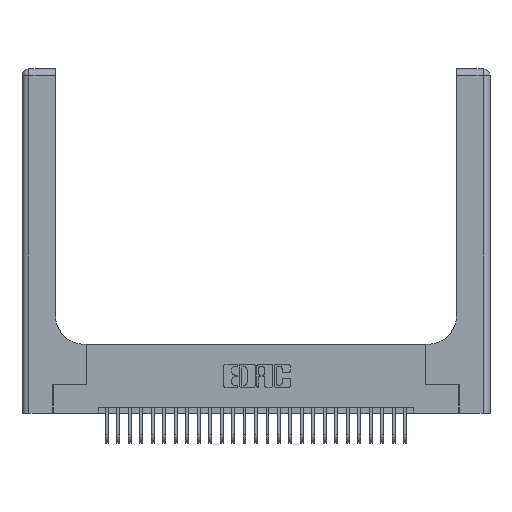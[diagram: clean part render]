
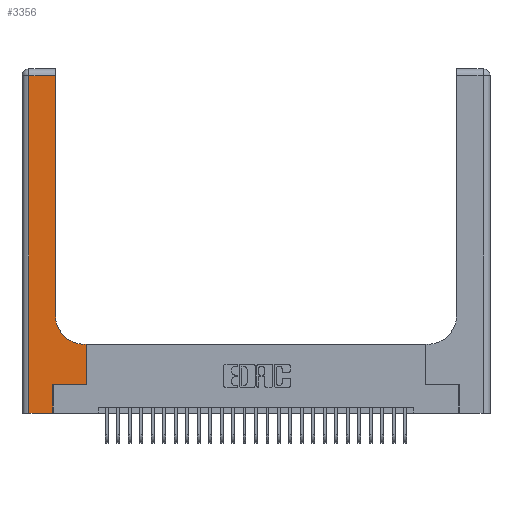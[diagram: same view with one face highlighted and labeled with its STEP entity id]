
A CAD part, top view. The second image highlights one B-rep face of the part: STEP entity #3356.
In plain terms, the highlighted planar face has unit normal (0, 0, 1).
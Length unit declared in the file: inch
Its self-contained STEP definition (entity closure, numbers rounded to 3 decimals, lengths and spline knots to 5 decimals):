
#152 = ORIENTED_EDGE ( 'NONE', *, *, #9684, .T. ) ;
#190 = EDGE_CURVE ( 'NONE', #2044, #9390, #6968, .T. ) ;
#1207 = ORIENTED_EDGE ( 'NONE', *, *, #14047, .T. ) ;
#1330 = VECTOR ( 'NONE', #9007, 39.37008 ) ;
#1758 = CARTESIAN_POINT ( 'NONE',  ( 0.2915, 3., 0.37 ) ) ;
#1813 = CARTESIAN_POINT ( 'NONE',  ( 0.269, 0.25, 0.37 ) ) ;
#2018 = EDGE_LOOP ( 'NONE', ( #13535, #4140, #25551, #152, #16556, #2170, #16359, #1207, #5405 ) ) ;
#2044 = VERTEX_POINT ( 'NONE', #18874 ) ;
#2170 = ORIENTED_EDGE ( 'NONE', *, *, #19964, .T. ) ;
#2260 = DIRECTION ( 'NONE',  ( 1., 0., 0. ) ) ;
#2372 = CARTESIAN_POINT ( 'NONE',  ( 0.269, 0.25, 0.37 ) ) ;
#2516 = CARTESIAN_POINT ( 'NONE',  ( 0.2915, 0.6, 0.37 ) ) ;
#3356 = ADVANCED_FACE ( 'NONE', ( #25059 ), #12335, .F. ) ;
#3654 = DIRECTION ( 'NONE',  ( 0., 0., -1. ) ) ;
#3860 = LINE ( 'NONE', #2372, #14624 ) ;
#3955 = DIRECTION ( 'NONE',  ( 0., 0., -1. ) ) ;
#4044 = DIRECTION ( 'NONE',  ( 0., -1., 0. ) ) ;
#4140 = ORIENTED_EDGE ( 'NONE', *, *, #23266, .T. ) ;
#5179 = LINE ( 'NONE', #14684, #26443 ) ;
#5287 = VERTEX_POINT ( 'NONE', #12602 ) ;
#5405 = ORIENTED_EDGE ( 'NONE', *, *, #15931, .T. ) ;
#5995 = AXIS2_PLACEMENT_3D ( 'NONE', #16468, #3654, #18598 ) ;
#6313 = VECTOR ( 'NONE', #21131, 39.37008 ) ;
#6968 = LINE ( 'NONE', #21126, #6313 ) ;
#9007 = DIRECTION ( 'NONE',  ( -1., 0., 0. ) ) ;
#9390 = VERTEX_POINT ( 'NONE', #22518 ) ;
#9440 = VERTEX_POINT ( 'NONE', #22958 ) ;
#9534 = DIRECTION ( 'NONE',  ( -1., 0., 0. ) ) ;
#9684 = EDGE_CURVE ( 'NONE', #12507, #16370, #10683, .T. ) ;
#10683 = LINE ( 'NONE', #25713, #26874 ) ;
#11013 = AXIS2_PLACEMENT_3D ( 'NONE', #16749, #3955, #18903 ) ;
#12335 = PLANE ( 'NONE',  #11013 ) ;
#12507 = VERTEX_POINT ( 'NONE', #18781 ) ;
#12533 = DIRECTION ( 'NONE',  ( 0., 1., 0. ) ) ;
#12602 = CARTESIAN_POINT ( 'NONE',  ( 0.06, 2.94, 0.37 ) ) ;
#12833 = LINE ( 'NONE', #2516, #1330 ) ;
#13219 = CARTESIAN_POINT ( 'NONE',  ( 0.2915, 2.94, 0.37 ) ) ;
#13535 = ORIENTED_EDGE ( 'NONE', *, *, #23711, .T. ) ;
#13866 = CARTESIAN_POINT ( 'NONE',  ( 0.2915, 0.85, 0.37 ) ) ;
#14047 = EDGE_CURVE ( 'NONE', #9390, #9440, #12833, .T. ) ;
#14624 = VECTOR ( 'NONE', #23636, 39.37008 ) ;
#14684 = CARTESIAN_POINT ( 'NONE',  ( 0.269, 0., 0.37 ) ) ;
#15686 = CIRCLE ( 'NONE', #5995, 0.25 ) ;
#15772 = VECTOR ( 'NONE', #9534, 39.37008 ) ;
#15931 = EDGE_CURVE ( 'NONE', #9440, #26290, #15686, .T. ) ;
#16359 = ORIENTED_EDGE ( 'NONE', *, *, #190, .T. ) ;
#16370 = VERTEX_POINT ( 'NONE', #24286 ) ;
#16441 = LINE ( 'NONE', #20114, #15772 ) ;
#16468 = CARTESIAN_POINT ( 'NONE',  ( 0.5415, 0.85, 0.37 ) ) ;
#16556 = ORIENTED_EDGE ( 'NONE', *, *, #20373, .T. ) ;
#16749 = CARTESIAN_POINT ( 'NONE',  ( 0., 3., 0.37 ) ) ;
#17307 = EDGE_CURVE ( 'NONE', #5287, #12507, #21218, .T. ) ;
#18598 = DIRECTION ( 'NONE',  ( 1., 0., 0. ) ) ;
#18781 = CARTESIAN_POINT ( 'NONE',  ( 0.06, 0., 0.37 ) ) ;
#18874 = CARTESIAN_POINT ( 'NONE',  ( 0.5585, 0.25, 0.37 ) ) ;
#18903 = DIRECTION ( 'NONE',  ( -1., 0., 0. ) ) ;
#19777 = VERTEX_POINT ( 'NONE', #1813 ) ;
#19964 = EDGE_CURVE ( 'NONE', #19777, #2044, #3860, .T. ) ;
#20114 = CARTESIAN_POINT ( 'NONE',  ( 0., 2.94, 0.37 ) ) ;
#20373 = EDGE_CURVE ( 'NONE', #16370, #19777, #5179, .T. ) ;
#21126 = CARTESIAN_POINT ( 'NONE',  ( 0.5585, 0.25, 0.37 ) ) ;
#21131 = DIRECTION ( 'NONE',  ( 0., 1., 0. ) ) ;
#21218 = LINE ( 'NONE', #25221, #21870 ) ;
#21870 = VECTOR ( 'NONE', #4044, 39.37008 ) ;
#22015 = LINE ( 'NONE', #1758, #27586 ) ;
#22518 = CARTESIAN_POINT ( 'NONE',  ( 0.5585, 0.6, 0.37 ) ) ;
#22958 = CARTESIAN_POINT ( 'NONE',  ( 0.5415, 0.6, 0.37 ) ) ;
#23266 = EDGE_CURVE ( 'NONE', #25074, #5287, #16441, .T. ) ;
#23636 = DIRECTION ( 'NONE',  ( 1., 0., 0. ) ) ;
#23711 = EDGE_CURVE ( 'NONE', #26290, #25074, #22015, .T. ) ;
#24286 = CARTESIAN_POINT ( 'NONE',  ( 0.269, 0., 0.37 ) ) ;
#25059 = FACE_OUTER_BOUND ( 'NONE', #2018, .T. ) ;
#25074 = VERTEX_POINT ( 'NONE', #13219 ) ;
#25221 = CARTESIAN_POINT ( 'NONE',  ( 0.06, 3., 0.37 ) ) ;
#25551 = ORIENTED_EDGE ( 'NONE', *, *, #17307, .T. ) ;
#25713 = CARTESIAN_POINT ( 'NONE',  ( 0., 0., 0.37 ) ) ;
#26290 = VERTEX_POINT ( 'NONE', #13866 ) ;
#26443 = VECTOR ( 'NONE', #27276, 39.37008 ) ;
#26874 = VECTOR ( 'NONE', #2260, 39.37008 ) ;
#27276 = DIRECTION ( 'NONE',  ( 0., 1., 0. ) ) ;
#27586 = VECTOR ( 'NONE', #12533, 39.37008 ) ;
